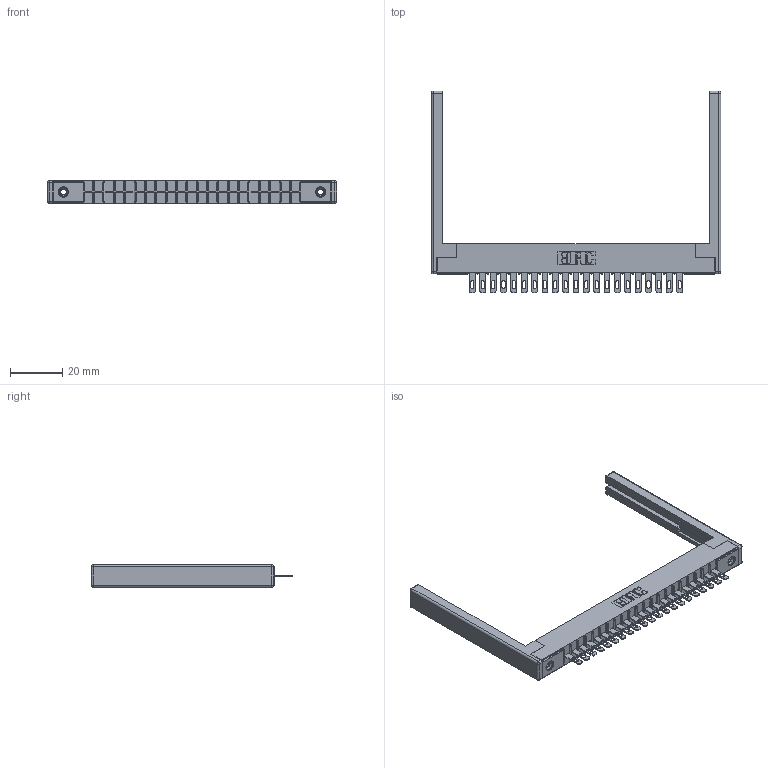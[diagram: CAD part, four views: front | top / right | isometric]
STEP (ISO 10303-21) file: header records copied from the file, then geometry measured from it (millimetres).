
FILE_DESCRIPTION (( 'STEP AP203' ), '1' );
FILE_NAME ('316-021-400-168.STEP', '2020-09-22T19:56:38', ( '' ), ( '' ), 'SwSTEP 2.0', 'SolidWorks 2020', '' );
FILE_SCHEMA (( 'CONFIG_CONTROL_DESIGN' ));
Length unit declared in the file: inch
Products named in the file (5): 307-220-068; 306 Part_.156 Dia; 345-250-001_345-250-001-102; 316-021-400-168; 306-290-001_100
Assembly tree (26 placements, depth 2):
  316-021-400-168
    306 Part_.156 Dia
    306-290-001_100  x21
    345-250-001_345-250-001-102  x2
    307-220-068  x2
Bounding box: 110.64 x 77.17 x 8.71 mm (x, y, z)
Volume: 12182.5 mm3; surface area: 15693.1 mm2
Topology: 26 solids, 26 shells, 1866 faces, 5221 edges, 3346 vertices
Faces by surface type: plane 1206, cylinder 552, sphere 92, cone 12, torus 4
Entity records: 25227 total; most frequent: CARTESIAN_POINT 4199, DIRECTION 4156, ORIENTED_EDGE 4152, EDGE_CURVE 2076, LINE 1606, VECTOR 1606, VERTEX_POINT 1318, AXIS2_PLACEMENT_3D 1275
